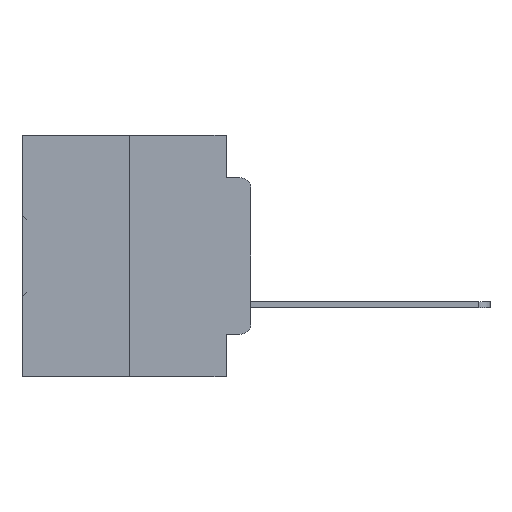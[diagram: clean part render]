
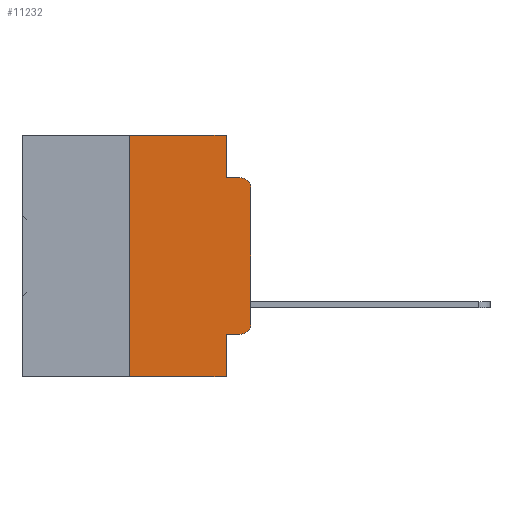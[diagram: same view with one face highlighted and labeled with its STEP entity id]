
A CAD part, left-side view. The second image highlights one B-rep face of the part: STEP entity #11232.
In plain terms, the highlighted planar face has unit normal (-1, 0, 0).
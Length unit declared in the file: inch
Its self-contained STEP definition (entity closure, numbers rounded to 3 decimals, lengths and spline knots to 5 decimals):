
#73 = VERTEX_POINT ( 'NONE', #14701 ) ;
#140 = VERTEX_POINT ( 'NONE', #16104 ) ;
#730 = ORIENTED_EDGE ( 'NONE', *, *, #6135, .F. ) ;
#996 = DIRECTION ( 'NONE',  ( 1., 0., 0. ) ) ;
#1436 = CARTESIAN_POINT ( 'NONE',  ( 0., 0., 0. ) ) ;
#1738 = CARTESIAN_POINT ( 'NONE',  ( 0., 0.051, 0. ) ) ;
#1755 = VECTOR ( 'NONE', #7451, 39.37008 ) ;
#1902 = LINE ( 'NONE', #28373, #29836 ) ;
#2174 = ORIENTED_EDGE ( 'NONE', *, *, #26687, .T. ) ;
#2442 = DIRECTION ( 'NONE',  ( 0., 0., -1. ) ) ;
#2996 = CARTESIAN_POINT ( 'NONE',  ( 0., 0.051, -0.4115 ) ) ;
#4434 = ORIENTED_EDGE ( 'NONE', *, *, #24866, .F. ) ;
#4814 = AXIS2_PLACEMENT_3D ( 'NONE', #35395, #19620, #2442 ) ;
#5049 = EDGE_LOOP ( 'NONE', ( #16767, #2174, #4434, #5200, #18223, #7032, #7137, #730, #7462, #8259 ) ) ;
#5200 = ORIENTED_EDGE ( 'NONE', *, *, #17747, .F. ) ;
#6135 = EDGE_CURVE ( 'NONE', #7304, #73, #24037, .T. ) ;
#7032 = ORIENTED_EDGE ( 'NONE', *, *, #8101, .F. ) ;
#7137 = ORIENTED_EDGE ( 'NONE', *, *, #33285, .T. ) ;
#7304 = VERTEX_POINT ( 'NONE', #2996 ) ;
#7314 = CARTESIAN_POINT ( 'NONE',  ( 0., 0.051, 0. ) ) ;
#7367 = VECTOR ( 'NONE', #24434, 39.37008 ) ;
#7451 = DIRECTION ( 'NONE',  ( 0., 0., 1. ) ) ;
#7462 = ORIENTED_EDGE ( 'NONE', *, *, #32588, .T. ) ;
#8101 = EDGE_CURVE ( 'NONE', #16786, #14230, #27707, .T. ) ;
#8246 = LINE ( 'NONE', #16647, #35447 ) ;
#8259 = ORIENTED_EDGE ( 'NONE', *, *, #23723, .T. ) ;
#8368 = DIRECTION ( 'NONE',  ( -1., 0., 0. ) ) ;
#9548 = LINE ( 'NONE', #1436, #1755 ) ;
#9827 = EDGE_CURVE ( 'NONE', #14230, #25091, #1902, .T. ) ;
#10993 = VERTEX_POINT ( 'NONE', #19525 ) ;
#11003 = LINE ( 'NONE', #19543, #30983 ) ;
#11079 = DIRECTION ( 'NONE',  ( 0., -1., 0. ) ) ;
#11232 = ADVANCED_FACE ( 'NONE', ( #33858 ), #31553, .F. ) ;
#11550 = CARTESIAN_POINT ( 'NONE',  ( 0., 0.25, 0. ) ) ;
#11668 = CIRCLE ( 'NONE', #18357, 0.02 ) ;
#12108 = DIRECTION ( 'NONE',  ( 0., -1., 0. ) ) ;
#12799 = VECTOR ( 'NONE', #12108, 39.37008 ) ;
#13712 = LINE ( 'NONE', #25696, #12799 ) ;
#14230 = VERTEX_POINT ( 'NONE', #11550 ) ;
#14701 = CARTESIAN_POINT ( 'NONE',  ( 0., 0.051, -0.5 ) ) ;
#15150 = LINE ( 'NONE', #1738, #7367 ) ;
#15240 = CARTESIAN_POINT ( 'NONE',  ( 0., 0.25, -0.5 ) ) ;
#15607 = CIRCLE ( 'NONE', #4814, 0.02 ) ;
#16104 = CARTESIAN_POINT ( 'NONE',  ( 0., 0.02, -0.4115 ) ) ;
#16647 = CARTESIAN_POINT ( 'NONE',  ( 0., 0.051, -0.4115 ) ) ;
#16767 = ORIENTED_EDGE ( 'NONE', *, *, #30244, .T. ) ;
#16786 = VERTEX_POINT ( 'NONE', #15240 ) ;
#17747 = EDGE_CURVE ( 'NONE', #25091, #20423, #15150, .T. ) ;
#17960 = DIRECTION ( 'NONE',  ( 0., 0., 1. ) ) ;
#18223 = ORIENTED_EDGE ( 'NONE', *, *, #9827, .F. ) ;
#18232 = CARTESIAN_POINT ( 'NONE',  ( 0., 0.473, 0. ) ) ;
#18357 = AXIS2_PLACEMENT_3D ( 'NONE', #24978, #8368, #27710 ) ;
#18725 = DIRECTION ( 'NONE',  ( 0., 0., -1. ) ) ;
#19366 = DIRECTION ( 'NONE',  ( 0., -1., 0. ) ) ;
#19460 = CARTESIAN_POINT ( 'NONE',  ( 0., 0.02, -0.0885 ) ) ;
#19525 = CARTESIAN_POINT ( 'NONE',  ( 0., 0., -0.3915 ) ) ;
#19543 = CARTESIAN_POINT ( 'NONE',  ( 0., 0.051, -0.0885 ) ) ;
#19620 = DIRECTION ( 'NONE',  ( -1., 0., 0. ) ) ;
#20423 = VERTEX_POINT ( 'NONE', #28380 ) ;
#21037 = DIRECTION ( 'NONE',  ( 0., 0., -1. ) ) ;
#23007 = DIRECTION ( 'NONE',  ( 0., -1., 0. ) ) ;
#23723 = EDGE_CURVE ( 'NONE', #140, #10993, #15607, .T. ) ;
#24037 = LINE ( 'NONE', #7314, #30316 ) ;
#24434 = DIRECTION ( 'NONE',  ( 0., 0., -1. ) ) ;
#24866 = EDGE_CURVE ( 'NONE', #20423, #33195, #11003, .T. ) ;
#24978 = CARTESIAN_POINT ( 'NONE',  ( 0., 0.02, -0.1085 ) ) ;
#25091 = VERTEX_POINT ( 'NONE', #25791 ) ;
#25379 = VECTOR ( 'NONE', #17960, 39.37008 ) ;
#25696 = CARTESIAN_POINT ( 'NONE',  ( 0., 0.473, -0.5 ) ) ;
#25791 = CARTESIAN_POINT ( 'NONE',  ( 0., 0.051, 0. ) ) ;
#26687 = EDGE_CURVE ( 'NONE', #33586, #33195, #11668, .T. ) ;
#27707 = LINE ( 'NONE', #33782, #25379 ) ;
#27710 = DIRECTION ( 'NONE',  ( 0., 0., -1. ) ) ;
#28231 = AXIS2_PLACEMENT_3D ( 'NONE', #18232, #996, #21037 ) ;
#28373 = CARTESIAN_POINT ( 'NONE',  ( 0., 0.473, 0. ) ) ;
#28380 = CARTESIAN_POINT ( 'NONE',  ( 0., 0.051, -0.0885 ) ) ;
#29836 = VECTOR ( 'NONE', #23007, 39.37008 ) ;
#30244 = EDGE_CURVE ( 'NONE', #10993, #33586, #9548, .T. ) ;
#30316 = VECTOR ( 'NONE', #18725, 39.37008 ) ;
#30983 = VECTOR ( 'NONE', #11079, 39.37008 ) ;
#31553 = PLANE ( 'NONE',  #28231 ) ;
#32588 = EDGE_CURVE ( 'NONE', #7304, #140, #8246, .T. ) ;
#33195 = VERTEX_POINT ( 'NONE', #19460 ) ;
#33285 = EDGE_CURVE ( 'NONE', #16786, #73, #13712, .T. ) ;
#33586 = VERTEX_POINT ( 'NONE', #34724 ) ;
#33782 = CARTESIAN_POINT ( 'NONE',  ( 0., 0.25, 0. ) ) ;
#33858 = FACE_OUTER_BOUND ( 'NONE', #5049, .T. ) ;
#34724 = CARTESIAN_POINT ( 'NONE',  ( 0., 0., -0.1085 ) ) ;
#35395 = CARTESIAN_POINT ( 'NONE',  ( 0., 0.02, -0.3915 ) ) ;
#35447 = VECTOR ( 'NONE', #19366, 39.37008 ) ;
